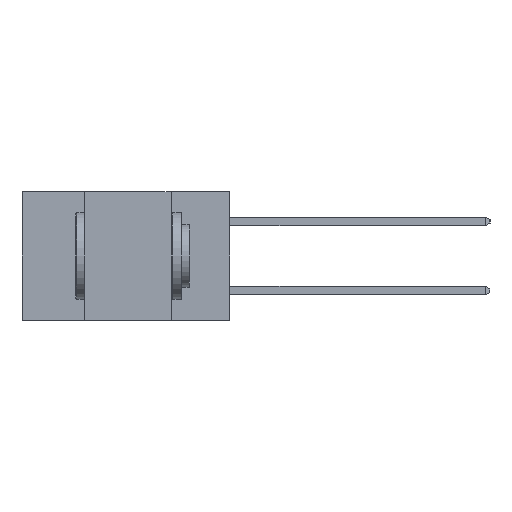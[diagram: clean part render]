
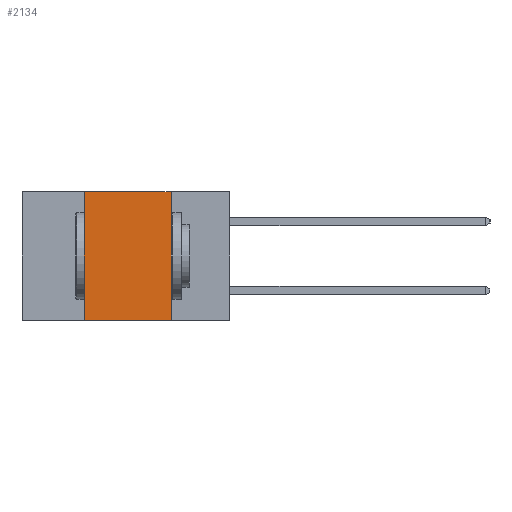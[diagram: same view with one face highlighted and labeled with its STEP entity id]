
A CAD part, left-side view. The second image highlights one B-rep face of the part: STEP entity #2134.
In plain terms, the highlighted planar face has unit normal (-1, 0, 0).
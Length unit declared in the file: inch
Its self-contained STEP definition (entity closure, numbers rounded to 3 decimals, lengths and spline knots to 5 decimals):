
#341 = EDGE_CURVE ( 'NONE', #17027, #7538, #11544, .T. ) ;
#572 = DIRECTION ( 'NONE',  ( 0., -1., 0. ) ) ;
#577 = AXIS2_PLACEMENT_3D ( 'NONE', #12969, #5905, #10749 ) ;
#948 = VECTOR ( 'NONE', #572, 39.37008 ) ;
#1730 = CARTESIAN_POINT ( 'NONE',  ( 0., 0.17, 0. ) ) ;
#2134 = ADVANCED_FACE ( 'NONE', ( #2780 ), #3982, .F. ) ;
#2780 = FACE_OUTER_BOUND ( 'NONE', #15098, .T. ) ;
#3047 = CARTESIAN_POINT ( 'NONE',  ( 0., 0.6, 0. ) ) ;
#3982 = PLANE ( 'NONE',  #577 ) ;
#5335 = VECTOR ( 'NONE', #9772, 39.37008 ) ;
#5676 = DIRECTION ( 'NONE',  ( 0., 0., 1. ) ) ;
#5905 = DIRECTION ( 'NONE',  ( 1., 0., 0. ) ) ;
#7315 = EDGE_CURVE ( 'NONE', #8548, #17027, #15292, .T. ) ;
#7538 = VERTEX_POINT ( 'NONE', #8596 ) ;
#8384 = VECTOR ( 'NONE', #5676, 39.37008 ) ;
#8548 = VERTEX_POINT ( 'NONE', #11409 ) ;
#8596 = CARTESIAN_POINT ( 'NONE',  ( 0., 0.17, 0. ) ) ;
#8991 = DIRECTION ( 'NONE',  ( 0., -1., 0. ) ) ;
#9489 = VERTEX_POINT ( 'NONE', #15879 ) ;
#9772 = DIRECTION ( 'NONE',  ( 0., 0., -1. ) ) ;
#10749 = DIRECTION ( 'NONE',  ( 0., 0., -1. ) ) ;
#10868 = ORIENTED_EDGE ( 'NONE', *, *, #14297, .F. ) ;
#10901 = ORIENTED_EDGE ( 'NONE', *, *, #341, .F. ) ;
#11111 = ORIENTED_EDGE ( 'NONE', *, *, #7315, .F. ) ;
#11212 = ORIENTED_EDGE ( 'NONE', *, *, #12864, .T. ) ;
#11409 = CARTESIAN_POINT ( 'NONE',  ( 0., 0.42, -0.37 ) ) ;
#11463 = LINE ( 'NONE', #1730, #5335 ) ;
#11519 = LINE ( 'NONE', #16685, #15022 ) ;
#11544 = LINE ( 'NONE', #3047, #948 ) ;
#12488 = CARTESIAN_POINT ( 'NONE',  ( 0., 0.42, 0. ) ) ;
#12864 = EDGE_CURVE ( 'NONE', #8548, #9489, #11519, .T. ) ;
#12969 = CARTESIAN_POINT ( 'NONE',  ( 0., 0.6, 0. ) ) ;
#14297 = EDGE_CURVE ( 'NONE', #7538, #9489, #11463, .T. ) ;
#15022 = VECTOR ( 'NONE', #8991, 39.37008 ) ;
#15098 = EDGE_LOOP ( 'NONE', ( #10868, #10901, #11111, #11212 ) ) ;
#15292 = LINE ( 'NONE', #12488, #8384 ) ;
#15879 = CARTESIAN_POINT ( 'NONE',  ( 0., 0.17, -0.37 ) ) ;
#16685 = CARTESIAN_POINT ( 'NONE',  ( 0., 0.6, -0.37 ) ) ;
#16745 = CARTESIAN_POINT ( 'NONE',  ( 0., 0.42, 0. ) ) ;
#17027 = VERTEX_POINT ( 'NONE', #16745 ) ;
